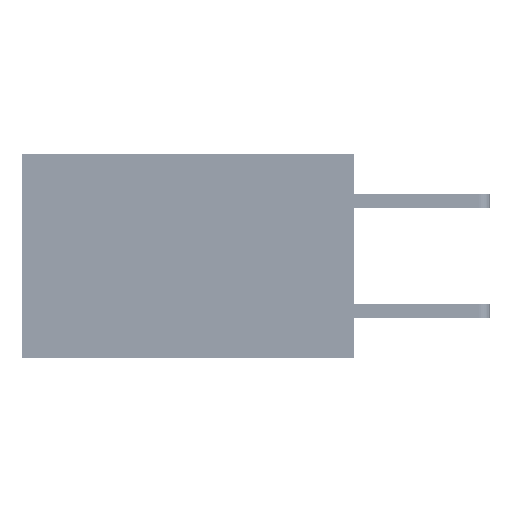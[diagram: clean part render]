
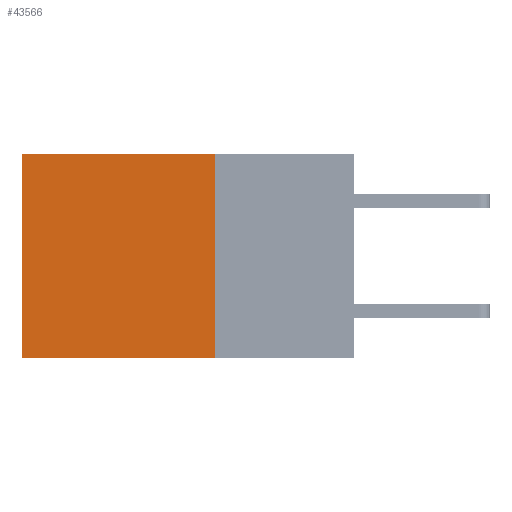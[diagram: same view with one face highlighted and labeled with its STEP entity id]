
A CAD part, left-side view. The second image highlights one B-rep face of the part: STEP entity #43566.
In plain terms, the highlighted planar face has unit normal (-1, 0, 0).
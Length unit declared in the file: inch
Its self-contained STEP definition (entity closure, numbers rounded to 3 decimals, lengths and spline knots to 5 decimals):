
#79 = VECTOR ( 'NONE', #8261, 39.37008 ) ;
#999 = VERTEX_POINT ( 'NONE', #8783 ) ;
#2213 = DIRECTION ( 'NONE',  ( 0., 0., -1. ) ) ;
#3646 = ORIENTED_EDGE ( 'NONE', *, *, #21320, .F. ) ;
#5318 = PLANE ( 'NONE',  #18950 ) ;
#6525 = VERTEX_POINT ( 'NONE', #24812 ) ;
#6752 = LINE ( 'NONE', #13380, #34846 ) ;
#6759 = VECTOR ( 'NONE', #17139, 39.37008 ) ;
#8261 = DIRECTION ( 'NONE',  ( 0., 0., -1. ) ) ;
#8783 = CARTESIAN_POINT ( 'NONE',  ( 0.2875, 0.6, -0.37 ) ) ;
#9036 = EDGE_CURVE ( 'NONE', #40519, #999, #29501, .T. ) ;
#12928 = EDGE_CURVE ( 'NONE', #22901, #40519, #32127, .T. ) ;
#13380 = CARTESIAN_POINT ( 'NONE',  ( 0.2875, 0.25, -0.37 ) ) ;
#16585 = CARTESIAN_POINT ( 'NONE',  ( 0.2875, 0.6, 0. ) ) ;
#17057 = EDGE_CURVE ( 'NONE', #6525, #999, #6752, .T. ) ;
#17139 = DIRECTION ( 'NONE',  ( 0., 0., -1. ) ) ;
#18900 = CARTESIAN_POINT ( 'NONE',  ( 0.2875, 0.25, 0. ) ) ;
#18950 = AXIS2_PLACEMENT_3D ( 'NONE', #32541, #35210, #2213 ) ;
#21320 = EDGE_CURVE ( 'NONE', #22901, #6525, #29989, .T. ) ;
#21721 = CARTESIAN_POINT ( 'NONE',  ( 0.2875, 0.25, 0. ) ) ;
#22389 = DIRECTION ( 'NONE',  ( 0., 1., 0. ) ) ;
#22901 = VERTEX_POINT ( 'NONE', #18900 ) ;
#23151 = DIRECTION ( 'NONE',  ( 0., 1., 0. ) ) ;
#24812 = CARTESIAN_POINT ( 'NONE',  ( 0.2875, 0.25, -0.37 ) ) ;
#25687 = FACE_OUTER_BOUND ( 'NONE', #27758, .T. ) ;
#26445 = CARTESIAN_POINT ( 'NONE',  ( 0.2875, 0.25, 0. ) ) ;
#27758 = EDGE_LOOP ( 'NONE', ( #34088, #42846, #3646, #32571 ) ) ;
#29501 = LINE ( 'NONE', #38606, #79 ) ;
#29989 = LINE ( 'NONE', #26445, #6759 ) ;
#32127 = LINE ( 'NONE', #21721, #35571 ) ;
#32541 = CARTESIAN_POINT ( 'NONE',  ( 0.2875, 0.25, 0. ) ) ;
#32571 = ORIENTED_EDGE ( 'NONE', *, *, #12928, .T. ) ;
#34088 = ORIENTED_EDGE ( 'NONE', *, *, #9036, .T. ) ;
#34846 = VECTOR ( 'NONE', #23151, 39.37008 ) ;
#35210 = DIRECTION ( 'NONE',  ( 1., 0., 0. ) ) ;
#35571 = VECTOR ( 'NONE', #22389, 39.37008 ) ;
#38606 = CARTESIAN_POINT ( 'NONE',  ( 0.2875, 0.6, 0. ) ) ;
#40519 = VERTEX_POINT ( 'NONE', #16585 ) ;
#42846 = ORIENTED_EDGE ( 'NONE', *, *, #17057, .F. ) ;
#43566 = ADVANCED_FACE ( 'NONE', ( #25687 ), #5318, .F. ) ;
